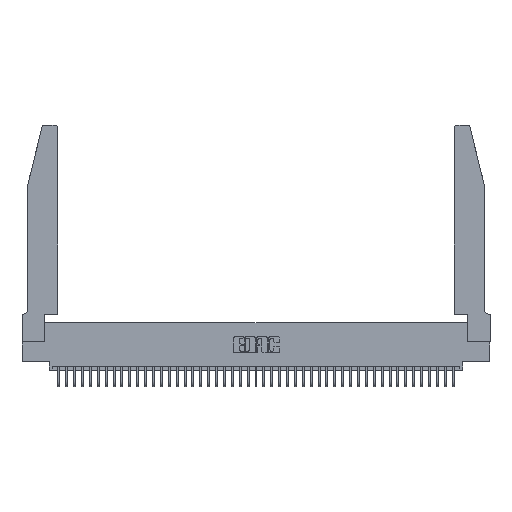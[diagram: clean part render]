
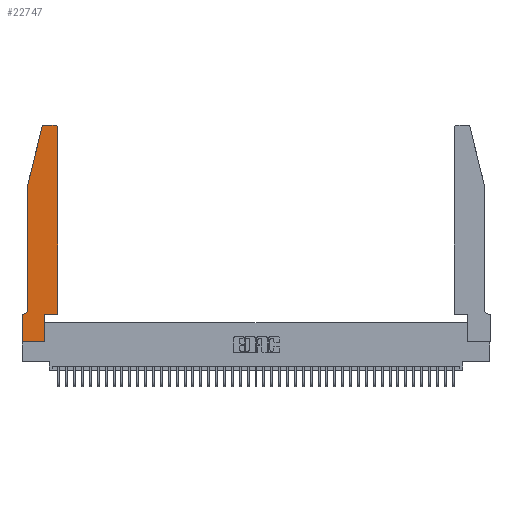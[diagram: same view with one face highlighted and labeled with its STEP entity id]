
A CAD part, top view. The second image highlights one B-rep face of the part: STEP entity #22747.
In plain terms, the highlighted planar face has unit normal (0, 0, 1).
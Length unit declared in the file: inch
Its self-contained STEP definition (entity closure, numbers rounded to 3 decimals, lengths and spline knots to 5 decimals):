
#370 = CIRCLE ( 'NONE', #24308, 0.03 ) ;
#1898 = DIRECTION ( 'NONE',  ( 0., 0., 1. ) ) ;
#1930 = VERTEX_POINT ( 'NONE', #17175 ) ;
#2519 = CARTESIAN_POINT ( 'NONE',  ( 0.0055, 0.35, 0.37 ) ) ;
#2873 = FACE_OUTER_BOUND ( 'NONE', #30761, .T. ) ;
#3442 = DIRECTION ( 'NONE',  ( 0., 0., 1. ) ) ;
#3506 = DIRECTION ( 'NONE',  ( 0., 0., -1. ) ) ;
#3571 = VERTEX_POINT ( 'NONE', #38453 ) ;
#4150 = VECTOR ( 'NONE', #7493, 39.37008 ) ;
#4440 = VERTEX_POINT ( 'NONE', #36758 ) ;
#5348 = LINE ( 'NONE', #26342, #12504 ) ;
#6248 = VERTEX_POINT ( 'NONE', #25915 ) ;
#6350 = CIRCLE ( 'NONE', #20554, 0.07 ) ;
#6774 = CARTESIAN_POINT ( 'NONE',  ( 0.0755, 2., 0.37 ) ) ;
#6812 = EDGE_CURVE ( 'NONE', #33152, #27888, #32966, .T. ) ;
#6818 = PLANE ( 'NONE',  #40360 ) ;
#6962 = DIRECTION ( 'NONE',  ( 1., 0., 0. ) ) ;
#7493 = DIRECTION ( 'NONE',  ( 1., 0., 0. ) ) ;
#7659 = VERTEX_POINT ( 'NONE', #19649 ) ;
#8576 = CARTESIAN_POINT ( 'NONE',  ( 0.2865, 0.35, 0.37 ) ) ;
#8632 = CARTESIAN_POINT ( 'NONE',  ( 0.284, 2.72, 0.37 ) ) ;
#9626 = EDGE_CURVE ( 'NONE', #4440, #3571, #15726, .T. ) ;
#9783 = VERTEX_POINT ( 'NONE', #20546 ) ;
#10382 = ORIENTED_EDGE ( 'NONE', *, *, #37195, .T. ) ;
#11090 = CARTESIAN_POINT ( 'NONE',  ( 0.4505, 2.72, 0.37 ) ) ;
#11270 = LINE ( 'NONE', #15198, #18385 ) ;
#12504 = VECTOR ( 'NONE', #33546, 39.37008 ) ;
#13547 = CARTESIAN_POINT ( 'NONE',  ( 0.4505, 0.35, 0.37 ) ) ;
#14570 = EDGE_CURVE ( 'NONE', #20059, #34532, #26440, .T. ) ;
#15198 = CARTESIAN_POINT ( 'NONE',  ( 0.2605, 2.75, 0.37 ) ) ;
#15726 = LINE ( 'NONE', #19478, #40919 ) ;
#16021 = ORIENTED_EDGE ( 'NONE', *, *, #16854, .T. ) ;
#16212 = CARTESIAN_POINT ( 'NONE',  ( 0.0755, 2., 0.37 ) ) ;
#16854 = EDGE_CURVE ( 'NONE', #24496, #1930, #370, .T. ) ;
#17175 = CARTESIAN_POINT ( 'NONE',  ( 0.4205, 2.75, 0.37 ) ) ;
#18255 = CARTESIAN_POINT ( 'NONE',  ( 0., 0.35, 0.37 ) ) ;
#18346 = CIRCLE ( 'NONE', #33533, 0.03 ) ;
#18385 = VECTOR ( 'NONE', #18731, 39.37008 ) ;
#18583 = EDGE_CURVE ( 'NONE', #6248, #43393, #6350, .T. ) ;
#18731 = DIRECTION ( 'NONE',  ( -1., 0., 0. ) ) ;
#19478 = CARTESIAN_POINT ( 'NONE',  ( 0.4505, 0.35, 0.37 ) ) ;
#19649 = CARTESIAN_POINT ( 'NONE',  ( 0.2865, 0., 0.37 ) ) ;
#20059 = VERTEX_POINT ( 'NONE', #32694 ) ;
#20291 = CARTESIAN_POINT ( 'NONE',  ( 0.0055, 0.42, 0.37 ) ) ;
#20398 = EDGE_CURVE ( 'NONE', #1930, #9783, #11270, .T. ) ;
#20478 = ORIENTED_EDGE ( 'NONE', *, *, #9626, .T. ) ;
#20546 = CARTESIAN_POINT ( 'NONE',  ( 0.284, 2.75, 0.37 ) ) ;
#20554 = AXIS2_PLACEMENT_3D ( 'NONE', #20291, #3506, #21165 ) ;
#20604 = CARTESIAN_POINT ( 'NONE',  ( 0.0755, 2., 0.37 ) ) ;
#20750 = DIRECTION ( 'NONE',  ( -0.239, -0.971, 0. ) ) ;
#21037 = CARTESIAN_POINT ( 'NONE',  ( 0., 0., 0.37 ) ) ;
#21063 = EDGE_CURVE ( 'NONE', #7659, #4440, #44189, .T. ) ;
#21165 = DIRECTION ( 'NONE',  ( -1., 0., 0. ) ) ;
#21398 = ORIENTED_EDGE ( 'NONE', *, *, #32845, .T. ) ;
#22747 = ADVANCED_FACE ( 'NONE', ( #2873 ), #6818, .T. ) ;
#24288 = DIRECTION ( 'NONE',  ( 0., 1., 0. ) ) ;
#24308 = AXIS2_PLACEMENT_3D ( 'NONE', #34420, #27536, #6962 ) ;
#24496 = VERTEX_POINT ( 'NONE', #11090 ) ;
#24958 = ORIENTED_EDGE ( 'NONE', *, *, #25919, .T. ) ;
#25125 = LINE ( 'NONE', #6774, #37202 ) ;
#25669 = LINE ( 'NONE', #13547, #38289 ) ;
#25912 = VECTOR ( 'NONE', #20750, 39.37008 ) ;
#25915 = CARTESIAN_POINT ( 'NONE',  ( 0.0755, 0.42, 0.37 ) ) ;
#25919 = EDGE_CURVE ( 'NONE', #43393, #33152, #5348, .T. ) ;
#26342 = CARTESIAN_POINT ( 'NONE',  ( 0.0755, 0.35, 0.37 ) ) ;
#26382 = ORIENTED_EDGE ( 'NONE', *, *, #14570, .T. ) ;
#26440 = LINE ( 'NONE', #20604, #25912 ) ;
#27274 = EDGE_CURVE ( 'NONE', #27888, #7659, #39231, .T. ) ;
#27536 = DIRECTION ( 'NONE',  ( 0., 0., 1. ) ) ;
#27888 = VERTEX_POINT ( 'NONE', #32007 ) ;
#27985 = CARTESIAN_POINT ( 'NONE',  ( 0., 0.35, 0.37 ) ) ;
#29653 = ORIENTED_EDGE ( 'NONE', *, *, #6812, .T. ) ;
#29958 = ORIENTED_EDGE ( 'NONE', *, *, #27274, .T. ) ;
#30761 = EDGE_LOOP ( 'NONE', ( #40163, #10382, #26382, #35054, #40863, #24958, #29653, #29958, #37588, #20478, #21398, #16021 ) ) ;
#32007 = CARTESIAN_POINT ( 'NONE',  ( 0., 0., 0.37 ) ) ;
#32121 = VECTOR ( 'NONE', #34321, 39.37008 ) ;
#32694 = CARTESIAN_POINT ( 'NONE',  ( 0.25487, 2.72718, 0.37 ) ) ;
#32845 = EDGE_CURVE ( 'NONE', #3571, #24496, #25669, .T. ) ;
#32876 = EDGE_CURVE ( 'NONE', #34532, #6248, #25125, .T. ) ;
#32966 = LINE ( 'NONE', #39740, #34606 ) ;
#33152 = VERTEX_POINT ( 'NONE', #18255 ) ;
#33533 = AXIS2_PLACEMENT_3D ( 'NONE', #8632, #1898, #36693 ) ;
#33546 = DIRECTION ( 'NONE',  ( -1., 0., 0. ) ) ;
#34321 = DIRECTION ( 'NONE',  ( 0., 1., 0. ) ) ;
#34420 = CARTESIAN_POINT ( 'NONE',  ( 0.4205, 2.72, 0.37 ) ) ;
#34532 = VERTEX_POINT ( 'NONE', #16212 ) ;
#34606 = VECTOR ( 'NONE', #36458, 39.37008 ) ;
#35054 = ORIENTED_EDGE ( 'NONE', *, *, #32876, .T. ) ;
#36458 = DIRECTION ( 'NONE',  ( 0., -1., 0. ) ) ;
#36693 = DIRECTION ( 'NONE',  ( 1., 0., 0. ) ) ;
#36758 = CARTESIAN_POINT ( 'NONE',  ( 0.2865, 0.35, 0.37 ) ) ;
#37195 = EDGE_CURVE ( 'NONE', #9783, #20059, #18346, .T. ) ;
#37202 = VECTOR ( 'NONE', #41252, 39.37008 ) ;
#37588 = ORIENTED_EDGE ( 'NONE', *, *, #21063, .T. ) ;
#38289 = VECTOR ( 'NONE', #24288, 39.37008 ) ;
#38453 = CARTESIAN_POINT ( 'NONE',  ( 0.4505, 0.35, 0.37 ) ) ;
#39231 = LINE ( 'NONE', #21037, #4150 ) ;
#39740 = CARTESIAN_POINT ( 'NONE',  ( 0., 0., 0.37 ) ) ;
#40163 = ORIENTED_EDGE ( 'NONE', *, *, #20398, .T. ) ;
#40360 = AXIS2_PLACEMENT_3D ( 'NONE', #27985, #3442, #45121 ) ;
#40863 = ORIENTED_EDGE ( 'NONE', *, *, #18583, .T. ) ;
#40919 = VECTOR ( 'NONE', #43798, 39.37008 ) ;
#41252 = DIRECTION ( 'NONE',  ( 0., -1., 0. ) ) ;
#43393 = VERTEX_POINT ( 'NONE', #2519 ) ;
#43798 = DIRECTION ( 'NONE',  ( 1., 0., 0. ) ) ;
#44189 = LINE ( 'NONE', #8576, #32121 ) ;
#45121 = DIRECTION ( 'NONE',  ( 1., 0., 0. ) ) ;
